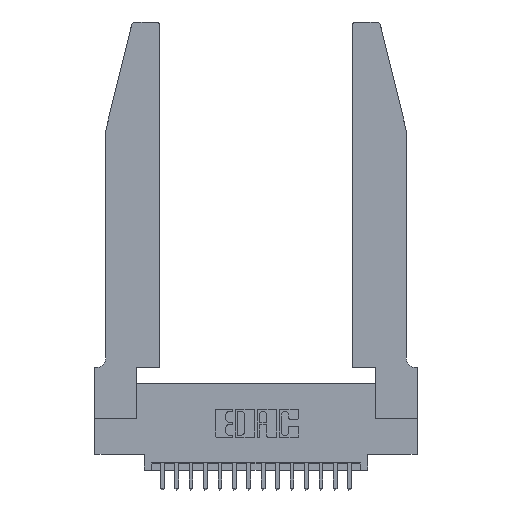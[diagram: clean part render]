
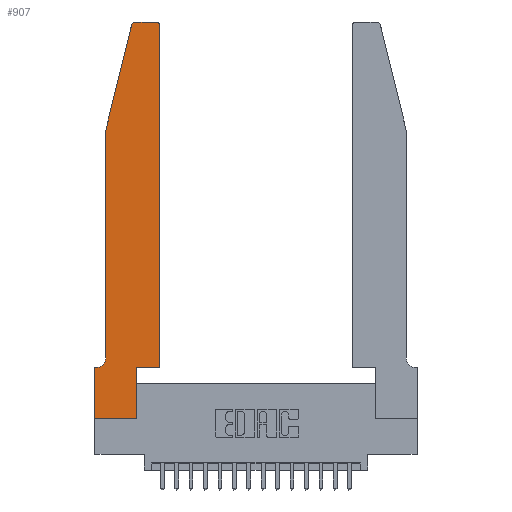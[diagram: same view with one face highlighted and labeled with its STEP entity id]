
A CAD part, top view. The second image highlights one B-rep face of the part: STEP entity #907.
In plain terms, the highlighted planar face has unit normal (0, 0, 1).
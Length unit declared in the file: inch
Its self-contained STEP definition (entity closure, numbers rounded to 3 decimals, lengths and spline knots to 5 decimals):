
#20 = EDGE_CURVE ( 'NONE', #131, #4589, #11039, .T. ) ;
#131 = VERTEX_POINT ( 'NONE', #13783 ) ;
#278 = DIRECTION ( 'NONE',  ( 1., 0., 0. ) ) ;
#555 = ORIENTED_EDGE ( 'NONE', *, *, #15798, .T. ) ;
#789 = DIRECTION ( 'NONE',  ( 0., 0., 1. ) ) ;
#907 = ADVANCED_FACE ( 'NONE', ( #17301 ), #3922, .T. ) ;
#1297 = DIRECTION ( 'NONE',  ( 0., -1., 0. ) ) ;
#1537 = AXIS2_PLACEMENT_3D ( 'NONE', #12562, #3511, #14059 ) ;
#1895 = EDGE_CURVE ( 'NONE', #7874, #13680, #18925, .T. ) ;
#1974 = VECTOR ( 'NONE', #8741, 39.37008 ) ;
#2083 = EDGE_CURVE ( 'NONE', #4589, #7874, #15677, .T. ) ;
#2478 = LINE ( 'NONE', #7218, #1974 ) ;
#2719 = CIRCLE ( 'NONE', #9494, 0.03 ) ;
#2761 = CARTESIAN_POINT ( 'NONE',  ( 0.0755, 0.35, 0.37 ) ) ;
#2887 = CARTESIAN_POINT ( 'NONE',  ( 0.4505, 0.35, 0.37 ) ) ;
#2915 = VECTOR ( 'NONE', #5490, 39.37008 ) ;
#2992 = VERTEX_POINT ( 'NONE', #15649 ) ;
#3256 = VERTEX_POINT ( 'NONE', #2887 ) ;
#3511 = DIRECTION ( 'NONE',  ( 0., 0., -1. ) ) ;
#3520 = DIRECTION ( 'NONE',  ( 0., 1., 0. ) ) ;
#3836 = AXIS2_PLACEMENT_3D ( 'NONE', #3940, #789, #278 ) ;
#3922 = PLANE ( 'NONE',  #3836 ) ;
#3940 = CARTESIAN_POINT ( 'NONE',  ( 0., 0.35, 0.37 ) ) ;
#4375 = CARTESIAN_POINT ( 'NONE',  ( 0., 0., 0.37 ) ) ;
#4589 = VERTEX_POINT ( 'NONE', #18012 ) ;
#4850 = ORIENTED_EDGE ( 'NONE', *, *, #1895, .T. ) ;
#4921 = EDGE_CURVE ( 'NONE', #10563, #16193, #6218, .T. ) ;
#5017 = VECTOR ( 'NONE', #7884, 39.37008 ) ;
#5194 = DIRECTION ( 'NONE',  ( 0., 0., 1. ) ) ;
#5215 = VECTOR ( 'NONE', #17813, 39.37008 ) ;
#5407 = CARTESIAN_POINT ( 'NONE',  ( 0., 0., 0.37 ) ) ;
#5490 = DIRECTION ( 'NONE',  ( 1., 0., 0. ) ) ;
#5994 = ORIENTED_EDGE ( 'NONE', *, *, #13480, .T. ) ;
#6218 = CIRCLE ( 'NONE', #12145, 0.03 ) ;
#6303 = ORIENTED_EDGE ( 'NONE', *, *, #19197, .T. ) ;
#6661 = CARTESIAN_POINT ( 'NONE',  ( 0.0755, 2., 0.37 ) ) ;
#7060 = DIRECTION ( 'NONE',  ( -1., 0., 0. ) ) ;
#7151 = LINE ( 'NONE', #7172, #18149 ) ;
#7172 = CARTESIAN_POINT ( 'NONE',  ( 0.2605, 2.75, 0.37 ) ) ;
#7218 = CARTESIAN_POINT ( 'NONE',  ( 0.4505, 0.35, 0.37 ) ) ;
#7313 = CARTESIAN_POINT ( 'NONE',  ( 0.25487, 2.72718, 0.37 ) ) ;
#7355 = ORIENTED_EDGE ( 'NONE', *, *, #10981, .T. ) ;
#7357 = CARTESIAN_POINT ( 'NONE',  ( 0.284, 2.72, 0.37 ) ) ;
#7377 = CARTESIAN_POINT ( 'NONE',  ( 0.0755, 2., 0.37 ) ) ;
#7746 = VECTOR ( 'NONE', #13651, 39.37008 ) ;
#7874 = VERTEX_POINT ( 'NONE', #5407 ) ;
#7884 = DIRECTION ( 'NONE',  ( 0., 1., 0. ) ) ;
#8497 = LINE ( 'NONE', #15555, #12896 ) ;
#8670 = EDGE_LOOP ( 'NONE', ( #555, #7355, #11408, #6303, #5994, #10126, #19035, #4850, #17189, #10714, #18978, #15926 ) ) ;
#8695 = DIRECTION ( 'NONE',  ( -1., 0., 0. ) ) ;
#8741 = DIRECTION ( 'NONE',  ( 1., 0., 0. ) ) ;
#8871 = DIRECTION ( 'NONE',  ( 1., 0., 0. ) ) ;
#9014 = CARTESIAN_POINT ( 'NONE',  ( 0.0755, 2., 0.37 ) ) ;
#9494 = AXIS2_PLACEMENT_3D ( 'NONE', #7357, #17795, #8871 ) ;
#10126 = ORIENTED_EDGE ( 'NONE', *, *, #20, .T. ) ;
#10563 = VERTEX_POINT ( 'NONE', #19500 ) ;
#10714 = ORIENTED_EDGE ( 'NONE', *, *, #17150, .T. ) ;
#10981 = EDGE_CURVE ( 'NONE', #2992, #14034, #2719, .T. ) ;
#11039 = LINE ( 'NONE', #2761, #15028 ) ;
#11408 = ORIENTED_EDGE ( 'NONE', *, *, #15881, .T. ) ;
#12094 = LINE ( 'NONE', #18327, #5017 ) ;
#12145 = AXIS2_PLACEMENT_3D ( 'NONE', #14179, #5194, #15718 ) ;
#12407 = CARTESIAN_POINT ( 'NONE',  ( 0., 0., 0.37 ) ) ;
#12438 = CARTESIAN_POINT ( 'NONE',  ( 0.0755, 0.42, 0.37 ) ) ;
#12562 = CARTESIAN_POINT ( 'NONE',  ( 0.0055, 0.42, 0.37 ) ) ;
#12726 = LINE ( 'NONE', #7377, #5215 ) ;
#12816 = CARTESIAN_POINT ( 'NONE',  ( 0.4205, 2.75, 0.37 ) ) ;
#12896 = VECTOR ( 'NONE', #3520, 39.37008 ) ;
#13480 = EDGE_CURVE ( 'NONE', #18763, #131, #15213, .T. ) ;
#13651 = DIRECTION ( 'NONE',  ( 0., -1., 0. ) ) ;
#13680 = VERTEX_POINT ( 'NONE', #13948 ) ;
#13783 = CARTESIAN_POINT ( 'NONE',  ( 0.0055, 0.35, 0.37 ) ) ;
#13948 = CARTESIAN_POINT ( 'NONE',  ( 0.2865, 0., 0.37 ) ) ;
#14034 = VERTEX_POINT ( 'NONE', #7313 ) ;
#14059 = DIRECTION ( 'NONE',  ( -1., 0., 0. ) ) ;
#14179 = CARTESIAN_POINT ( 'NONE',  ( 0.4205, 2.72, 0.37 ) ) ;
#14772 = VECTOR ( 'NONE', #1297, 39.37008 ) ;
#14836 = EDGE_CURVE ( 'NONE', #3256, #10563, #12094, .T. ) ;
#15028 = VECTOR ( 'NONE', #7060, 39.37008 ) ;
#15213 = CIRCLE ( 'NONE', #1537, 0.07 ) ;
#15555 = CARTESIAN_POINT ( 'NONE',  ( 0.2865, 0.35, 0.37 ) ) ;
#15649 = CARTESIAN_POINT ( 'NONE',  ( 0.284, 2.75, 0.37 ) ) ;
#15677 = LINE ( 'NONE', #4375, #7746 ) ;
#15718 = DIRECTION ( 'NONE',  ( 1., 0., 0. ) ) ;
#15798 = EDGE_CURVE ( 'NONE', #16193, #2992, #7151, .T. ) ;
#15881 = EDGE_CURVE ( 'NONE', #14034, #18113, #12726, .T. ) ;
#15926 = ORIENTED_EDGE ( 'NONE', *, *, #4921, .T. ) ;
#16193 = VERTEX_POINT ( 'NONE', #12816 ) ;
#16573 = CARTESIAN_POINT ( 'NONE',  ( 0.2865, 0.35, 0.37 ) ) ;
#17150 = EDGE_CURVE ( 'NONE', #17310, #3256, #2478, .T. ) ;
#17189 = ORIENTED_EDGE ( 'NONE', *, *, #19598, .T. ) ;
#17301 = FACE_OUTER_BOUND ( 'NONE', #8670, .T. ) ;
#17310 = VERTEX_POINT ( 'NONE', #16573 ) ;
#17795 = DIRECTION ( 'NONE',  ( 0., 0., 1. ) ) ;
#17813 = DIRECTION ( 'NONE',  ( -0.239, -0.971, 0. ) ) ;
#18012 = CARTESIAN_POINT ( 'NONE',  ( 0., 0.35, 0.37 ) ) ;
#18113 = VERTEX_POINT ( 'NONE', #6661 ) ;
#18149 = VECTOR ( 'NONE', #8695, 39.37008 ) ;
#18327 = CARTESIAN_POINT ( 'NONE',  ( 0.4505, 0.35, 0.37 ) ) ;
#18763 = VERTEX_POINT ( 'NONE', #12438 ) ;
#18925 = LINE ( 'NONE', #12407, #2915 ) ;
#18978 = ORIENTED_EDGE ( 'NONE', *, *, #14836, .T. ) ;
#19035 = ORIENTED_EDGE ( 'NONE', *, *, #2083, .T. ) ;
#19197 = EDGE_CURVE ( 'NONE', #18113, #18763, #19674, .T. ) ;
#19500 = CARTESIAN_POINT ( 'NONE',  ( 0.4505, 2.72, 0.37 ) ) ;
#19598 = EDGE_CURVE ( 'NONE', #13680, #17310, #8497, .T. ) ;
#19674 = LINE ( 'NONE', #9014, #14772 ) ;
